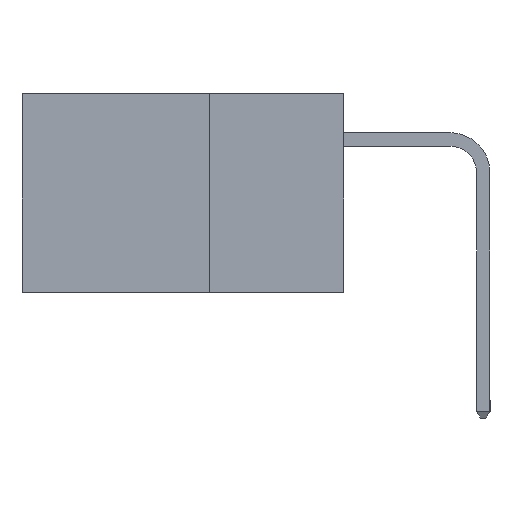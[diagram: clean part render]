
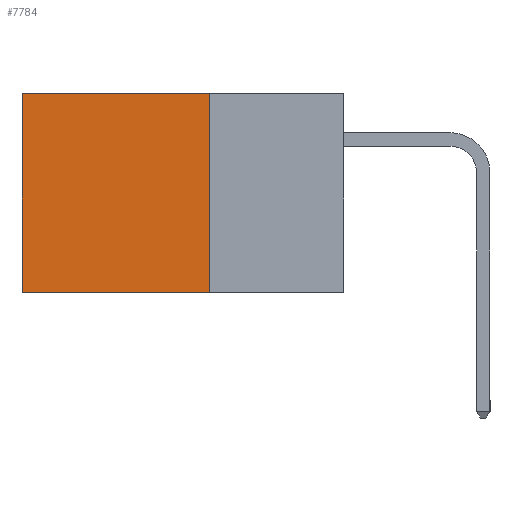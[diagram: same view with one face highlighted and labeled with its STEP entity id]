
A CAD part, left-side view. The second image highlights one B-rep face of the part: STEP entity #7784.
In plain terms, the highlighted planar face has unit normal (-1, 0, 0).
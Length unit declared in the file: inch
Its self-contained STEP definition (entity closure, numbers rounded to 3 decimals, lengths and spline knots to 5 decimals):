
#561 = DIRECTION ( 'NONE',  ( 0., 1., 0. ) ) ;
#834 = ORIENTED_EDGE ( 'NONE', *, *, #13358, .T. ) ;
#3789 = EDGE_CURVE ( 'NONE', #23702, #21617, #4946, .T. ) ;
#3928 = CARTESIAN_POINT ( 'NONE',  ( 0.2615, 0.25, -0.37 ) ) ;
#4421 = CARTESIAN_POINT ( 'NONE',  ( 0.2615, 0.6, -0.37 ) ) ;
#4946 = LINE ( 'NONE', #20148, #9471 ) ;
#6563 = DIRECTION ( 'NONE',  ( 0., 0., -1. ) ) ;
#7083 = LINE ( 'NONE', #3928, #11561 ) ;
#7784 = ADVANCED_FACE ( 'NONE', ( #22270 ), #14904, .F. ) ;
#8618 = AXIS2_PLACEMENT_3D ( 'NONE', #14955, #14868, #14847 ) ;
#9390 = CARTESIAN_POINT ( 'NONE',  ( 0.2615, 0.25, -0.37 ) ) ;
#9471 = VECTOR ( 'NONE', #20140, 39.37008 ) ;
#10155 = CARTESIAN_POINT ( 'NONE',  ( 0.2615, 0.25, 0. ) ) ;
#10340 = CARTESIAN_POINT ( 'NONE',  ( 0.2615, 0.6, -0.37 ) ) ;
#11561 = VECTOR ( 'NONE', #19385, 39.37008 ) ;
#12740 = LINE ( 'NONE', #23720, #16072 ) ;
#12742 = EDGE_CURVE ( 'NONE', #23702, #12872, #12740, .T. ) ;
#12872 = VERTEX_POINT ( 'NONE', #22522 ) ;
#13358 = EDGE_CURVE ( 'NONE', #12872, #23721, #22108, .T. ) ;
#14847 = DIRECTION ( 'NONE',  ( 0., 0., -1. ) ) ;
#14868 = DIRECTION ( 'NONE',  ( 1., 0., 0. ) ) ;
#14904 = PLANE ( 'NONE',  #8618 ) ;
#14955 = CARTESIAN_POINT ( 'NONE',  ( 0.2615, 0.25, -0.37 ) ) ;
#15062 = ORIENTED_EDGE ( 'NONE', *, *, #12742, .T. ) ;
#16072 = VECTOR ( 'NONE', #561, 39.37008 ) ;
#16874 = EDGE_LOOP ( 'NONE', ( #834, #23477, #17023, #15062 ) ) ;
#16933 = VECTOR ( 'NONE', #6563, 39.37008 ) ;
#17023 = ORIENTED_EDGE ( 'NONE', *, *, #3789, .F. ) ;
#19385 = DIRECTION ( 'NONE',  ( 0., 1., 0. ) ) ;
#20140 = DIRECTION ( 'NONE',  ( 0., 0., -1. ) ) ;
#20148 = CARTESIAN_POINT ( 'NONE',  ( 0.2615, 0.25, -0.37 ) ) ;
#21064 = EDGE_CURVE ( 'NONE', #21617, #23721, #7083, .T. ) ;
#21617 = VERTEX_POINT ( 'NONE', #9390 ) ;
#22108 = LINE ( 'NONE', #10340, #16933 ) ;
#22270 = FACE_OUTER_BOUND ( 'NONE', #16874, .T. ) ;
#22522 = CARTESIAN_POINT ( 'NONE',  ( 0.2615, 0.6, 0. ) ) ;
#23477 = ORIENTED_EDGE ( 'NONE', *, *, #21064, .F. ) ;
#23702 = VERTEX_POINT ( 'NONE', #10155 ) ;
#23720 = CARTESIAN_POINT ( 'NONE',  ( 0.2615, 0.25, 0. ) ) ;
#23721 = VERTEX_POINT ( 'NONE', #4421 ) ;
